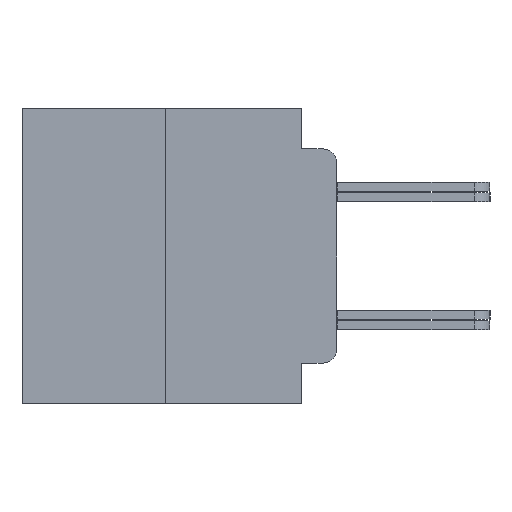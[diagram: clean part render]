
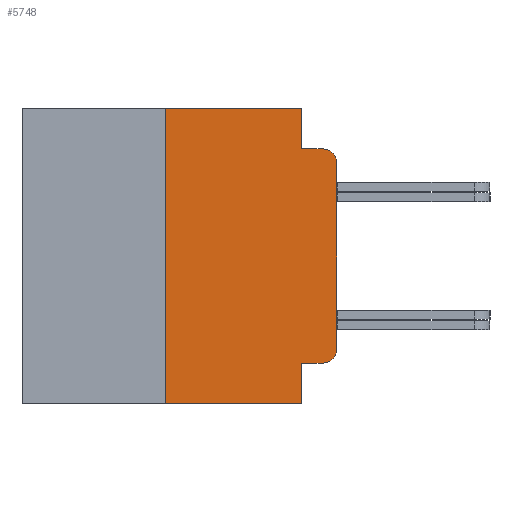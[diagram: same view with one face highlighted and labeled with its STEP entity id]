
A CAD part, left-side view. The second image highlights one B-rep face of the part: STEP entity #5748.
In plain terms, the highlighted planar face has unit normal (-1, 0, 0).
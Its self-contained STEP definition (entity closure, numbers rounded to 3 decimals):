
#219 = ORIENTED_EDGE ( 'NONE', *, *, #13031, .F. ) ;
#829 = ORIENTED_EDGE ( 'NONE', *, *, #12770, .T. ) ;
#1267 = VECTOR ( 'NONE', #8093, 1000. ) ;
#1566 = CIRCLE ( 'NONE', #3610, 0.508 ) ;
#1673 = CARTESIAN_POINT ( 'NONE',  ( -75.603, 6.35, 5.486 ) ) ;
#1884 = VECTOR ( 'NONE', #9579, 1000. ) ;
#1912 = LINE ( 'NONE', #14093, #23428 ) ;
#2247 = AXIS2_PLACEMENT_3D ( 'NONE', #17157, #12486, #28546 ) ;
#3511 = VECTOR ( 'NONE', #6673, 1000. ) ;
#3610 = AXIS2_PLACEMENT_3D ( 'NONE', #16709, #21342, #28294 ) ;
#4071 = CARTESIAN_POINT ( 'NONE',  ( -75.603, 1.295, -3.975 ) ) ;
#4439 = VERTEX_POINT ( 'NONE', #14622 ) ;
#4470 = ORIENTED_EDGE ( 'NONE', *, *, #20363, .F. ) ;
#4678 = CARTESIAN_POINT ( 'NONE',  ( -75.603, 11.684, 5.486 ) ) ;
#5144 = VERTEX_POINT ( 'NONE', #6900 ) ;
#5558 = EDGE_CURVE ( 'NONE', #11813, #14062, #13437, .T. ) ;
#5748 = ADVANCED_FACE ( 'NONE', ( #7302 ), #16000, .F. ) ;
#6098 = DIRECTION ( 'NONE',  ( 0., 0., -1. ) ) ;
#6673 = DIRECTION ( 'NONE',  ( 0., -1., 0. ) ) ;
#6841 = VERTEX_POINT ( 'NONE', #22089 ) ;
#6900 = CARTESIAN_POINT ( 'NONE',  ( -75.603, 0., -3.467 ) ) ;
#7106 = ORIENTED_EDGE ( 'NONE', *, *, #26232, .T. ) ;
#7206 = LINE ( 'NONE', #22183, #10097 ) ;
#7302 = FACE_OUTER_BOUND ( 'NONE', #28897, .T. ) ;
#7746 = LINE ( 'NONE', #16706, #21019 ) ;
#8093 = DIRECTION ( 'NONE',  ( 0., -1., 0. ) ) ;
#8159 = CARTESIAN_POINT ( 'NONE',  ( -75.603, 1.295, 5.486 ) ) ;
#8519 = VERTEX_POINT ( 'NONE', #18603 ) ;
#9482 = ORIENTED_EDGE ( 'NONE', *, *, #12507, .T. ) ;
#9571 = ORIENTED_EDGE ( 'NONE', *, *, #21357, .F. ) ;
#9579 = DIRECTION ( 'NONE',  ( 0., 0., 1. ) ) ;
#10097 = VECTOR ( 'NONE', #26644, 1000. ) ;
#11524 = DIRECTION ( 'NONE',  ( 0., 0., -1. ) ) ;
#11711 = DIRECTION ( 'NONE',  ( 1., 0., 0. ) ) ;
#11813 = VERTEX_POINT ( 'NONE', #24379 ) ;
#12149 = EDGE_CURVE ( 'NONE', #4439, #16521, #1912, .T. ) ;
#12340 = ORIENTED_EDGE ( 'NONE', *, *, #12149, .F. ) ;
#12486 = DIRECTION ( 'NONE',  ( -1., 0., 0. ) ) ;
#12507 = EDGE_CURVE ( 'NONE', #11813, #23006, #26299, .T. ) ;
#12518 = CARTESIAN_POINT ( 'NONE',  ( -75.603, 1.295, -5.486 ) ) ;
#12770 = EDGE_CURVE ( 'NONE', #5144, #6841, #28450, .T. ) ;
#13031 = EDGE_CURVE ( 'NONE', #16521, #25067, #7206, .T. ) ;
#13437 = LINE ( 'NONE', #29100, #24565 ) ;
#14062 = VERTEX_POINT ( 'NONE', #12518 ) ;
#14093 = CARTESIAN_POINT ( 'NONE',  ( -75.603, 6.35, -5.486 ) ) ;
#14622 = CARTESIAN_POINT ( 'NONE',  ( -75.603, 6.35, -5.486 ) ) ;
#14991 = ORIENTED_EDGE ( 'NONE', *, *, #27391, .T. ) ;
#14999 = CARTESIAN_POINT ( 'NONE',  ( -75.603, 11.684, -5.486 ) ) ;
#15612 = LINE ( 'NONE', #14999, #1267 ) ;
#16000 = PLANE ( 'NONE',  #23839 ) ;
#16521 = VERTEX_POINT ( 'NONE', #1673 ) ;
#16706 = CARTESIAN_POINT ( 'NONE',  ( -75.603, 1.295, 0. ) ) ;
#16709 = CARTESIAN_POINT ( 'NONE',  ( -75.603, 0.508, -3.467 ) ) ;
#17099 = LINE ( 'NONE', #27263, #3511 ) ;
#17157 = CARTESIAN_POINT ( 'NONE',  ( -75.603, 0.508, 3.467 ) ) ;
#18603 = CARTESIAN_POINT ( 'NONE',  ( -75.603, 0.508, 3.975 ) ) ;
#19500 = VERTEX_POINT ( 'NONE', #19644 ) ;
#19644 = CARTESIAN_POINT ( 'NONE',  ( -75.603, 1.295, 3.975 ) ) ;
#20363 = EDGE_CURVE ( 'NONE', #19500, #8519, #17099, .T. ) ;
#21019 = VECTOR ( 'NONE', #21637, 1000. ) ;
#21342 = DIRECTION ( 'NONE',  ( -1., 0., 0. ) ) ;
#21357 = EDGE_CURVE ( 'NONE', #25067, #19500, #7746, .T. ) ;
#21637 = DIRECTION ( 'NONE',  ( 0., 0., -1. ) ) ;
#22089 = CARTESIAN_POINT ( 'NONE',  ( -75.603, 0., 3.467 ) ) ;
#22183 = CARTESIAN_POINT ( 'NONE',  ( -75.603, 11.684, 5.486 ) ) ;
#23006 = VERTEX_POINT ( 'NONE', #28756 ) ;
#23428 = VECTOR ( 'NONE', #25670, 1000. ) ;
#23556 = CIRCLE ( 'NONE', #2247, 0.508 ) ;
#23839 = AXIS2_PLACEMENT_3D ( 'NONE', #4678, #11711, #11524 ) ;
#24379 = CARTESIAN_POINT ( 'NONE',  ( -75.603, 1.295, -3.975 ) ) ;
#24565 = VECTOR ( 'NONE', #6098, 1000. ) ;
#24725 = DIRECTION ( 'NONE',  ( 0., -1., 0. ) ) ;
#25067 = VERTEX_POINT ( 'NONE', #8159 ) ;
#25184 = ORIENTED_EDGE ( 'NONE', *, *, #5558, .F. ) ;
#25234 = ORIENTED_EDGE ( 'NONE', *, *, #25652, .T. ) ;
#25652 = EDGE_CURVE ( 'NONE', #4439, #14062, #15612, .T. ) ;
#25670 = DIRECTION ( 'NONE',  ( 0., 0., 1. ) ) ;
#26232 = EDGE_CURVE ( 'NONE', #6841, #8519, #23556, .T. ) ;
#26299 = LINE ( 'NONE', #4071, #27743 ) ;
#26644 = DIRECTION ( 'NONE',  ( 0., -1., 0. ) ) ;
#27263 = CARTESIAN_POINT ( 'NONE',  ( -75.603, 1.295, 3.975 ) ) ;
#27391 = EDGE_CURVE ( 'NONE', #23006, #5144, #1566, .T. ) ;
#27743 = VECTOR ( 'NONE', #24725, 1000. ) ;
#27859 = CARTESIAN_POINT ( 'NONE',  ( -75.603, 0., 5.486 ) ) ;
#28294 = DIRECTION ( 'NONE',  ( 0., 0., -1. ) ) ;
#28450 = LINE ( 'NONE', #27859, #1884 ) ;
#28546 = DIRECTION ( 'NONE',  ( 0., 0., -1. ) ) ;
#28756 = CARTESIAN_POINT ( 'NONE',  ( -75.603, 0.508, -3.975 ) ) ;
#28897 = EDGE_LOOP ( 'NONE', ( #9482, #14991, #829, #7106, #4470, #9571, #219, #12340, #25234, #25184 ) ) ;
#29100 = CARTESIAN_POINT ( 'NONE',  ( -75.603, 1.295, 0. ) ) ;
